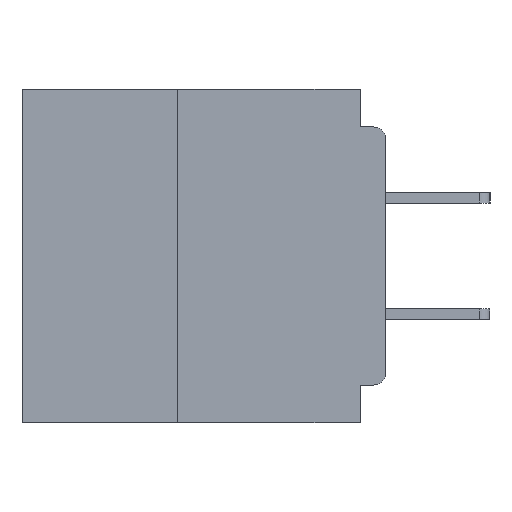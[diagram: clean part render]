
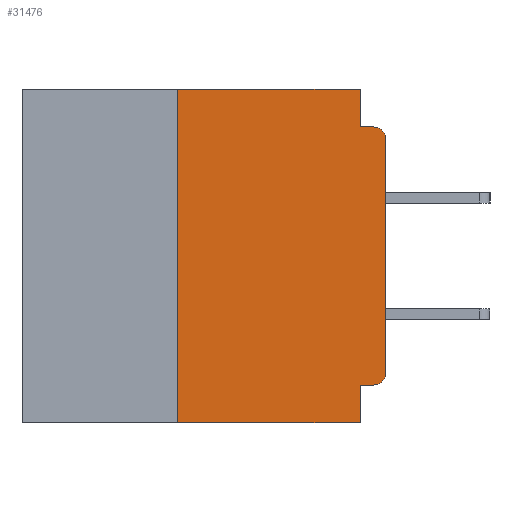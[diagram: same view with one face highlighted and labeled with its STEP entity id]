
A CAD part, left-side view. The second image highlights one B-rep face of the part: STEP entity #31476.
In plain terms, the highlighted planar face has unit normal (-1, 0, 0).
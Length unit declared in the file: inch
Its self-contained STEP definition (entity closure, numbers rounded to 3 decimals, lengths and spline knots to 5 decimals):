
#1156 = AXIS2_PLACEMENT_3D ( 'NONE', #41821, #10873, #47028 ) ;
#3276 = FACE_OUTER_BOUND ( 'NONE', #52588, .T. ) ;
#8160 = EDGE_CURVE ( 'NONE', #34244, #14379, #22118, .T. ) ;
#10018 = VERTEX_POINT ( 'NONE', #49830 ) ;
#10114 = CARTESIAN_POINT ( 'NONE',  ( 0., 0.031, -0.4 ) ) ;
#10719 = ORIENTED_EDGE ( 'NONE', *, *, #24350, .F. ) ;
#10873 = DIRECTION ( 'NONE',  ( -1., 0., 0. ) ) ;
#10956 = VECTOR ( 'NONE', #26346, 39.37008 ) ;
#11925 = VERTEX_POINT ( 'NONE', #25915 ) ;
#12033 = VECTOR ( 'NONE', #59630, 39.37008 ) ;
#12594 = LINE ( 'NONE', #21135, #10956 ) ;
#13654 = LINE ( 'NONE', #64609, #12033 ) ;
#14379 = VERTEX_POINT ( 'NONE', #65002 ) ;
#16108 = VERTEX_POINT ( 'NONE', #16616 ) ;
#16138 = EDGE_CURVE ( 'NONE', #32403, #29312, #34404, .T. ) ;
#16616 = CARTESIAN_POINT ( 'NONE',  ( 0., 0.031, -0.355 ) ) ;
#16841 = CARTESIAN_POINT ( 'NONE',  ( 0., 0.437, 0. ) ) ;
#17427 = AXIS2_PLACEMENT_3D ( 'NONE', #21450, #26677, #62853 ) ;
#17532 = CARTESIAN_POINT ( 'NONE',  ( 0., 0.031, 0. ) ) ;
#17712 = CIRCLE ( 'NONE', #1156, 0.015 ) ;
#18460 = CARTESIAN_POINT ( 'NONE',  ( 0., 0.25, -0.4 ) ) ;
#19647 = EDGE_CURVE ( 'NONE', #20613, #16108, #13654, .T. ) ;
#20442 = VECTOR ( 'NONE', #43488, 39.37008 ) ;
#20613 = VERTEX_POINT ( 'NONE', #31278 ) ;
#20751 = CARTESIAN_POINT ( 'NONE',  ( 0., 0.25, -0.4 ) ) ;
#21135 = CARTESIAN_POINT ( 'NONE',  ( 0., 0., 0. ) ) ;
#21450 = CARTESIAN_POINT ( 'NONE',  ( 0., 0.437, 0. ) ) ;
#22118 = LINE ( 'NONE', #23838, #49618 ) ;
#22800 = CARTESIAN_POINT ( 'NONE',  ( 0., 0.031, -0.045 ) ) ;
#23838 = CARTESIAN_POINT ( 'NONE',  ( 0., 0.437, -0.4 ) ) ;
#24350 = EDGE_CURVE ( 'NONE', #60087, #47201, #51363, .T. ) ;
#25915 = CARTESIAN_POINT ( 'NONE',  ( 0., 0., -0.06 ) ) ;
#26238 = CARTESIAN_POINT ( 'NONE',  ( 0., 0.015, -0.06 ) ) ;
#26268 = DIRECTION ( 'NONE',  ( 0., -1., 0. ) ) ;
#26346 = DIRECTION ( 'NONE',  ( 0., 0., 1. ) ) ;
#26677 = DIRECTION ( 'NONE',  ( 1., 0., 0. ) ) ;
#27281 = DIRECTION ( 'NONE',  ( 0., -1., 0. ) ) ;
#29312 = VERTEX_POINT ( 'NONE', #39987 ) ;
#30378 = EDGE_CURVE ( 'NONE', #29312, #60087, #34211, .T. ) ;
#31278 = CARTESIAN_POINT ( 'NONE',  ( 0., 0.015, -0.355 ) ) ;
#31462 = DIRECTION ( 'NONE',  ( 0., 0., -1. ) ) ;
#31476 = ADVANCED_FACE ( 'NONE', ( #3276 ), #52432, .F. ) ;
#32239 = EDGE_CURVE ( 'NONE', #34244, #32403, #63957, .T. ) ;
#32403 = VERTEX_POINT ( 'NONE', #60917 ) ;
#33092 = CIRCLE ( 'NONE', #44336, 0.015 ) ;
#33165 = EDGE_CURVE ( 'NONE', #11925, #47201, #33092, .T. ) ;
#34211 = LINE ( 'NONE', #17532, #20442 ) ;
#34244 = VERTEX_POINT ( 'NONE', #20751 ) ;
#34256 = VECTOR ( 'NONE', #66872, 39.37008 ) ;
#34257 = ORIENTED_EDGE ( 'NONE', *, *, #16138, .F. ) ;
#34345 = ORIENTED_EDGE ( 'NONE', *, *, #54317, .T. ) ;
#34404 = LINE ( 'NONE', #16841, #46500 ) ;
#34851 = EDGE_CURVE ( 'NONE', #10018, #11925, #12594, .T. ) ;
#35664 = ORIENTED_EDGE ( 'NONE', *, *, #33165, .T. ) ;
#35870 = LINE ( 'NONE', #10114, #34256 ) ;
#36095 = EDGE_CURVE ( 'NONE', #16108, #14379, #35870, .T. ) ;
#38691 = ORIENTED_EDGE ( 'NONE', *, *, #30378, .F. ) ;
#39228 = VECTOR ( 'NONE', #26268, 39.37008 ) ;
#39987 = CARTESIAN_POINT ( 'NONE',  ( 0., 0.031, 0. ) ) ;
#41316 = ORIENTED_EDGE ( 'NONE', *, *, #36095, .F. ) ;
#41821 = CARTESIAN_POINT ( 'NONE',  ( 0., 0.015, -0.34 ) ) ;
#42612 = ORIENTED_EDGE ( 'NONE', *, *, #34851, .T. ) ;
#43488 = DIRECTION ( 'NONE',  ( 0., 0., -1. ) ) ;
#43757 = ORIENTED_EDGE ( 'NONE', *, *, #32239, .F. ) ;
#44157 = DIRECTION ( 'NONE',  ( 0., -1., 0. ) ) ;
#44336 = AXIS2_PLACEMENT_3D ( 'NONE', #26238, #62410, #31462 ) ;
#46500 = VECTOR ( 'NONE', #27281, 39.37008 ) ;
#47028 = DIRECTION ( 'NONE',  ( 0., 0., -1. ) ) ;
#47201 = VERTEX_POINT ( 'NONE', #58869 ) ;
#47332 = ORIENTED_EDGE ( 'NONE', *, *, #8160, .T. ) ;
#48562 = VECTOR ( 'NONE', #54600, 39.37008 ) ;
#49618 = VECTOR ( 'NONE', #44157, 39.37008 ) ;
#49830 = CARTESIAN_POINT ( 'NONE',  ( 0., 0., -0.34 ) ) ;
#51363 = LINE ( 'NONE', #57239, #39228 ) ;
#52432 = PLANE ( 'NONE',  #17427 ) ;
#52588 = EDGE_LOOP ( 'NONE', ( #42612, #35664, #10719, #38691, #34257, #43757, #47332, #41316, #58989, #34345 ) ) ;
#54317 = EDGE_CURVE ( 'NONE', #20613, #10018, #17712, .T. ) ;
#54600 = DIRECTION ( 'NONE',  ( 0., 0., 1. ) ) ;
#57239 = CARTESIAN_POINT ( 'NONE',  ( 0., 0., -0.045 ) ) ;
#58869 = CARTESIAN_POINT ( 'NONE',  ( 0., 0.015, -0.045 ) ) ;
#58989 = ORIENTED_EDGE ( 'NONE', *, *, #19647, .F. ) ;
#59630 = DIRECTION ( 'NONE',  ( 0., 1., 0. ) ) ;
#60087 = VERTEX_POINT ( 'NONE', #22800 ) ;
#60917 = CARTESIAN_POINT ( 'NONE',  ( 0., 0.25, 0. ) ) ;
#62410 = DIRECTION ( 'NONE',  ( -1., 0., 0. ) ) ;
#62853 = DIRECTION ( 'NONE',  ( 0., 0., -1. ) ) ;
#63957 = LINE ( 'NONE', #18460, #48562 ) ;
#64609 = CARTESIAN_POINT ( 'NONE',  ( 0., 0., -0.355 ) ) ;
#65002 = CARTESIAN_POINT ( 'NONE',  ( 0., 0.031, -0.4 ) ) ;
#66872 = DIRECTION ( 'NONE',  ( 0., 0., -1. ) ) ;
